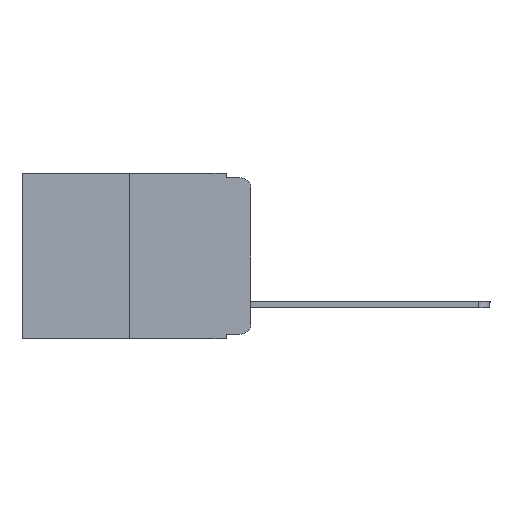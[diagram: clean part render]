
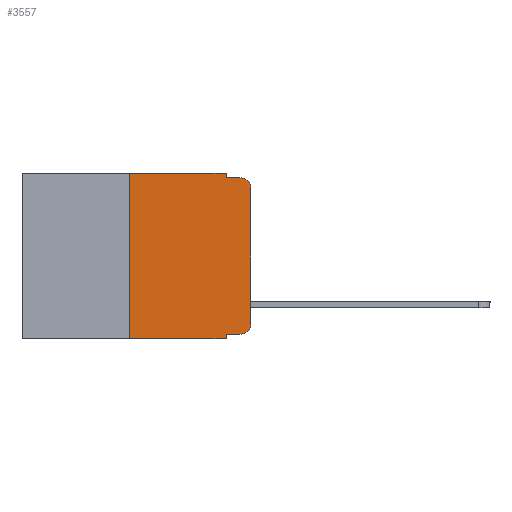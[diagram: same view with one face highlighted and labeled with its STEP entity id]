
A CAD part, left-side view. The second image highlights one B-rep face of the part: STEP entity #3557.
In plain terms, the highlighted planar face has unit normal (-1, 0, 0).
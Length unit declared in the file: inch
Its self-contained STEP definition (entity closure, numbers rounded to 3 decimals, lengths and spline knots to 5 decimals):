
#9 = DIRECTION ( 'NONE',  ( 0., 0., -1. ) ) ;
#19 = VECTOR ( 'NONE', #11424, 39.37008 ) ;
#283 = LINE ( 'NONE', #5850, #19 ) ;
#1164 = DIRECTION ( 'NONE',  ( 0., 0., -1. ) ) ;
#1450 = LINE ( 'NONE', #15416, #7769 ) ;
#1503 = CARTESIAN_POINT ( 'NONE',  ( 0., 0.051, -0.343 ) ) ;
#1751 = ORIENTED_EDGE ( 'NONE', *, *, #2971, .F. ) ;
#1921 = PLANE ( 'NONE',  #11343 ) ;
#1926 = AXIS2_PLACEMENT_3D ( 'NONE', #2753, #5576, #9 ) ;
#2055 = DIRECTION ( 'NONE',  ( 0., -1., 0. ) ) ;
#2206 = ORIENTED_EDGE ( 'NONE', *, *, #3206, .T. ) ;
#2447 = EDGE_CURVE ( 'NONE', #6001, #12996, #17998, .T. ) ;
#2531 = LINE ( 'NONE', #8086, #11328 ) ;
#2609 = CARTESIAN_POINT ( 'NONE',  ( 0., 0.02, -0.333 ) ) ;
#2753 = CARTESIAN_POINT ( 'NONE',  ( 0., 0.02, -0.03 ) ) ;
#2761 = VERTEX_POINT ( 'NONE', #16156 ) ;
#2787 = VECTOR ( 'NONE', #7531, 39.37008 ) ;
#2930 = DIRECTION ( 'NONE',  ( 1., 0., 0. ) ) ;
#2971 = EDGE_CURVE ( 'NONE', #8974, #4017, #2531, .T. ) ;
#3020 = CARTESIAN_POINT ( 'NONE',  ( 0., 0.02, -0.01 ) ) ;
#3050 = EDGE_CURVE ( 'NONE', #6001, #11952, #14029, .T. ) ;
#3206 = EDGE_CURVE ( 'NONE', #4643, #11952, #8799, .T. ) ;
#3443 = CARTESIAN_POINT ( 'NONE',  ( 0., 0.051, -0.01 ) ) ;
#3557 = ADVANCED_FACE ( 'NONE', ( #14254 ), #1921, .F. ) ;
#4017 = VERTEX_POINT ( 'NONE', #3443 ) ;
#4035 = VECTOR ( 'NONE', #5896, 39.37008 ) ;
#4259 = DIRECTION ( 'NONE',  ( -1., 0., 0. ) ) ;
#4629 = EDGE_CURVE ( 'NONE', #13652, #8974, #283, .T. ) ;
#4643 = VERTEX_POINT ( 'NONE', #8498 ) ;
#4872 = LINE ( 'NONE', #6072, #7021 ) ;
#5154 = LINE ( 'NONE', #10718, #2787 ) ;
#5576 = DIRECTION ( 'NONE',  ( -1., 0., 0. ) ) ;
#5627 = CARTESIAN_POINT ( 'NONE',  ( 0., 0.051, 0. ) ) ;
#5744 = ORIENTED_EDGE ( 'NONE', *, *, #2447, .T. ) ;
#5850 = CARTESIAN_POINT ( 'NONE',  ( 0., 0.473, 0. ) ) ;
#5896 = DIRECTION ( 'NONE',  ( 0., 0., -1. ) ) ;
#5940 = CARTESIAN_POINT ( 'NONE',  ( 0., 0.473, 0. ) ) ;
#6001 = VERTEX_POINT ( 'NONE', #14714 ) ;
#6072 = CARTESIAN_POINT ( 'NONE',  ( 0., 0.051, -0.01 ) ) ;
#6768 = EDGE_CURVE ( 'NONE', #4017, #9407, #4872, .T. ) ;
#6792 = ORIENTED_EDGE ( 'NONE', *, *, #4629, .F. ) ;
#6808 = EDGE_LOOP ( 'NONE', ( #16702, #11888, #17943, #1751, #6792, #7550, #2206, #7934, #5744, #17462 ) ) ;
#7021 = VECTOR ( 'NONE', #2055, 39.37008 ) ;
#7081 = CARTESIAN_POINT ( 'NONE',  ( 0., 0.02, -0.313 ) ) ;
#7531 = DIRECTION ( 'NONE',  ( 0., 0., 1. ) ) ;
#7550 = ORIENTED_EDGE ( 'NONE', *, *, #12796, .F. ) ;
#7763 = CIRCLE ( 'NONE', #1926, 0.02 ) ;
#7769 = VECTOR ( 'NONE', #16709, 39.37008 ) ;
#7934 = ORIENTED_EDGE ( 'NONE', *, *, #3050, .F. ) ;
#8086 = CARTESIAN_POINT ( 'NONE',  ( 0., 0.051, 0. ) ) ;
#8498 = CARTESIAN_POINT ( 'NONE',  ( 0., 0.25, -0.343 ) ) ;
#8799 = LINE ( 'NONE', #14390, #17772 ) ;
#8974 = VERTEX_POINT ( 'NONE', #13995 ) ;
#9390 = DIRECTION ( 'NONE',  ( 0., -1., 0. ) ) ;
#9407 = VERTEX_POINT ( 'NONE', #3020 ) ;
#10160 = VERTEX_POINT ( 'NONE', #17616 ) ;
#10718 = CARTESIAN_POINT ( 'NONE',  ( 0., 0.25, 0. ) ) ;
#11328 = VECTOR ( 'NONE', #1164, 39.37008 ) ;
#11343 = AXIS2_PLACEMENT_3D ( 'NONE', #5940, #2930, #11513 ) ;
#11424 = DIRECTION ( 'NONE',  ( 0., -1., 0. ) ) ;
#11450 = EDGE_CURVE ( 'NONE', #12996, #10160, #14717, .T. ) ;
#11513 = DIRECTION ( 'NONE',  ( 0., 0., -1. ) ) ;
#11823 = DIRECTION ( 'NONE',  ( 0., -1., 0. ) ) ;
#11888 = ORIENTED_EDGE ( 'NONE', *, *, #13404, .T. ) ;
#11952 = VERTEX_POINT ( 'NONE', #1503 ) ;
#12374 = VECTOR ( 'NONE', #9390, 39.37008 ) ;
#12796 = EDGE_CURVE ( 'NONE', #4643, #13652, #5154, .T. ) ;
#12996 = VERTEX_POINT ( 'NONE', #2609 ) ;
#13404 = EDGE_CURVE ( 'NONE', #2761, #9407, #7763, .T. ) ;
#13652 = VERTEX_POINT ( 'NONE', #14882 ) ;
#13681 = CARTESIAN_POINT ( 'NONE',  ( 0., 0.051, -0.333 ) ) ;
#13736 = EDGE_CURVE ( 'NONE', #10160, #2761, #1450, .T. ) ;
#13995 = CARTESIAN_POINT ( 'NONE',  ( 0., 0.051, 0. ) ) ;
#14029 = LINE ( 'NONE', #5627, #4035 ) ;
#14254 = FACE_OUTER_BOUND ( 'NONE', #6808, .T. ) ;
#14390 = CARTESIAN_POINT ( 'NONE',  ( 0., 0.473, -0.343 ) ) ;
#14714 = CARTESIAN_POINT ( 'NONE',  ( 0., 0.051, -0.333 ) ) ;
#14717 = CIRCLE ( 'NONE', #17382, 0.02 ) ;
#14882 = CARTESIAN_POINT ( 'NONE',  ( 0., 0.25, 0. ) ) ;
#15416 = CARTESIAN_POINT ( 'NONE',  ( 0., 0., 0. ) ) ;
#16156 = CARTESIAN_POINT ( 'NONE',  ( 0., 0., -0.03 ) ) ;
#16515 = DIRECTION ( 'NONE',  ( 0., 0., -1. ) ) ;
#16702 = ORIENTED_EDGE ( 'NONE', *, *, #13736, .T. ) ;
#16709 = DIRECTION ( 'NONE',  ( 0., 0., 1. ) ) ;
#17382 = AXIS2_PLACEMENT_3D ( 'NONE', #7081, #4259, #16515 ) ;
#17462 = ORIENTED_EDGE ( 'NONE', *, *, #11450, .T. ) ;
#17616 = CARTESIAN_POINT ( 'NONE',  ( 0., 0., -0.313 ) ) ;
#17772 = VECTOR ( 'NONE', #11823, 39.37008 ) ;
#17943 = ORIENTED_EDGE ( 'NONE', *, *, #6768, .F. ) ;
#17998 = LINE ( 'NONE', #13681, #12374 ) ;
